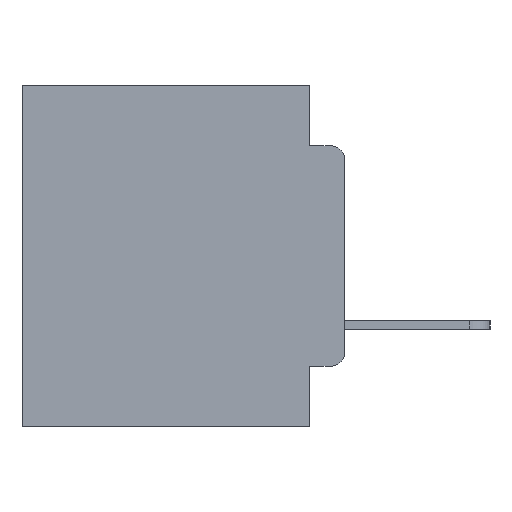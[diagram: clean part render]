
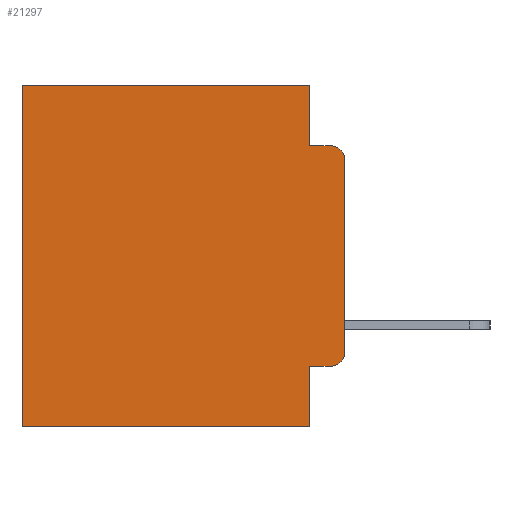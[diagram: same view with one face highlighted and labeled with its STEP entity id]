
A CAD part, left-side view. The second image highlights one B-rep face of the part: STEP entity #21297.
In plain terms, the highlighted planar face has unit normal (-1, 0, 0).
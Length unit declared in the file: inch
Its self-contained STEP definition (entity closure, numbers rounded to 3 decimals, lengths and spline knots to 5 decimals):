
#231 = DIRECTION ( 'NONE',  ( 0., 1., 0. ) ) ;
#335 = ORIENTED_EDGE ( 'NONE', *, *, #5590, .F. ) ;
#476 = VECTOR ( 'NONE', #7063, 39.37008 ) ;
#842 = VERTEX_POINT ( 'NONE', #13256 ) ;
#956 = VECTOR ( 'NONE', #26244, 39.37008 ) ;
#1646 = LINE ( 'NONE', #15390, #10868 ) ;
#1993 = VERTEX_POINT ( 'NONE', #24854 ) ;
#2411 = DIRECTION ( 'NONE',  ( -1., 0., 0. ) ) ;
#2981 = CIRCLE ( 'NONE', #24995, 0.02 ) ;
#3426 = DIRECTION ( 'NONE',  ( 1., 0., 0. ) ) ;
#3777 = CARTESIAN_POINT ( 'NONE',  ( 0.298, 0.02, -0.1085 ) ) ;
#4353 = CARTESIAN_POINT ( 'NONE',  ( 0.298, 0.051, -0.4115 ) ) ;
#4535 = LINE ( 'NONE', #24744, #9102 ) ;
#4929 = CARTESIAN_POINT ( 'NONE',  ( 0.298, 0.051, 0. ) ) ;
#5284 = ORIENTED_EDGE ( 'NONE', *, *, #26712, .T. ) ;
#5350 = LINE ( 'NONE', #10343, #20196 ) ;
#5549 = ORIENTED_EDGE ( 'NONE', *, *, #22947, .T. ) ;
#5590 = EDGE_CURVE ( 'NONE', #842, #29036, #24272, .T. ) ;
#6640 = FACE_OUTER_BOUND ( 'NONE', #8624, .T. ) ;
#6986 = ORIENTED_EDGE ( 'NONE', *, *, #18214, .F. ) ;
#7063 = DIRECTION ( 'NONE',  ( 0., 0., -1. ) ) ;
#7308 = ORIENTED_EDGE ( 'NONE', *, *, #20765, .T. ) ;
#7462 = VECTOR ( 'NONE', #9378, 39.37008 ) ;
#7862 = EDGE_CURVE ( 'NONE', #10213, #24569, #27596, .T. ) ;
#8111 = AXIS2_PLACEMENT_3D ( 'NONE', #20575, #2411, #24910 ) ;
#8624 = EDGE_LOOP ( 'NONE', ( #14654, #5549, #335, #27455, #5284, #23179, #21137, #6986, #7308, #28510 ) ) ;
#9102 = VECTOR ( 'NONE', #27571, 39.37008 ) ;
#9378 = DIRECTION ( 'NONE',  ( 0., 0., -1. ) ) ;
#10139 = CARTESIAN_POINT ( 'NONE',  ( 0.298, 0., 0. ) ) ;
#10213 = VERTEX_POINT ( 'NONE', #28214 ) ;
#10343 = CARTESIAN_POINT ( 'NONE',  ( 0.298, 0., -0.5 ) ) ;
#10488 = CARTESIAN_POINT ( 'NONE',  ( 0.298, 0.02, -0.0885 ) ) ;
#10587 = DIRECTION ( 'NONE',  ( -1., 0., 0. ) ) ;
#10801 = CARTESIAN_POINT ( 'NONE',  ( 0.298, 0.051, 0. ) ) ;
#10868 = VECTOR ( 'NONE', #26693, 39.37008 ) ;
#11604 = VERTEX_POINT ( 'NONE', #4353 ) ;
#13084 = EDGE_CURVE ( 'NONE', #14661, #842, #4535, .T. ) ;
#13256 = CARTESIAN_POINT ( 'NONE',  ( 0.298, 0.051, -0.0885 ) ) ;
#13297 = DIRECTION ( 'NONE',  ( 0., 0., -1. ) ) ;
#14654 = ORIENTED_EDGE ( 'NONE', *, *, #24735, .F. ) ;
#14661 = VERTEX_POINT ( 'NONE', #10801 ) ;
#15390 = CARTESIAN_POINT ( 'NONE',  ( 0.298, 0.051, -0.4115 ) ) ;
#16493 = EDGE_CURVE ( 'NONE', #24280, #1993, #28730, .T. ) ;
#17251 = AXIS2_PLACEMENT_3D ( 'NONE', #10139, #3426, #13297 ) ;
#17669 = VERTEX_POINT ( 'NONE', #21399 ) ;
#18214 = EDGE_CURVE ( 'NONE', #11604, #21427, #28245, .T. ) ;
#19735 = DIRECTION ( 'NONE',  ( 0., 0., -1. ) ) ;
#20196 = VECTOR ( 'NONE', #21965, 39.37008 ) ;
#20575 = CARTESIAN_POINT ( 'NONE',  ( 0.298, 0.02, -0.3915 ) ) ;
#20765 = EDGE_CURVE ( 'NONE', #11604, #10213, #1646, .T. ) ;
#21137 = ORIENTED_EDGE ( 'NONE', *, *, #24698, .F. ) ;
#21297 = ADVANCED_FACE ( 'NONE', ( #6640 ), #23628, .F. ) ;
#21381 = CARTESIAN_POINT ( 'NONE',  ( 0.298, 0.473, 0. ) ) ;
#21399 = CARTESIAN_POINT ( 'NONE',  ( 0.298, 0., -0.1085 ) ) ;
#21427 = VERTEX_POINT ( 'NONE', #25463 ) ;
#21949 = VECTOR ( 'NONE', #26487, 39.37008 ) ;
#21965 = DIRECTION ( 'NONE',  ( 0., 1., 0. ) ) ;
#22063 = CARTESIAN_POINT ( 'NONE',  ( 0.298, 0., 0. ) ) ;
#22947 = EDGE_CURVE ( 'NONE', #17669, #29036, #2981, .T. ) ;
#23179 = ORIENTED_EDGE ( 'NONE', *, *, #16493, .T. ) ;
#23628 = PLANE ( 'NONE',  #17251 ) ;
#24272 = LINE ( 'NONE', #28393, #956 ) ;
#24280 = VERTEX_POINT ( 'NONE', #21381 ) ;
#24569 = VERTEX_POINT ( 'NONE', #28527 ) ;
#24698 = EDGE_CURVE ( 'NONE', #21427, #1993, #5350, .T. ) ;
#24735 = EDGE_CURVE ( 'NONE', #17669, #24569, #25800, .T. ) ;
#24744 = CARTESIAN_POINT ( 'NONE',  ( 0.298, 0.051, 0. ) ) ;
#24854 = CARTESIAN_POINT ( 'NONE',  ( 0.298, 0.473, -0.5 ) ) ;
#24910 = DIRECTION ( 'NONE',  ( 0., 0., -1. ) ) ;
#24994 = CARTESIAN_POINT ( 'NONE',  ( 0.298, 0., 0. ) ) ;
#24995 = AXIS2_PLACEMENT_3D ( 'NONE', #3777, #10587, #19735 ) ;
#25463 = CARTESIAN_POINT ( 'NONE',  ( 0.298, 0.051, -0.5 ) ) ;
#25800 = LINE ( 'NONE', #22063, #21949 ) ;
#26244 = DIRECTION ( 'NONE',  ( 0., -1., 0. ) ) ;
#26389 = VECTOR ( 'NONE', #231, 39.37008 ) ;
#26487 = DIRECTION ( 'NONE',  ( 0., 0., -1. ) ) ;
#26693 = DIRECTION ( 'NONE',  ( 0., -1., 0. ) ) ;
#26712 = EDGE_CURVE ( 'NONE', #14661, #24280, #28136, .T. ) ;
#27125 = CARTESIAN_POINT ( 'NONE',  ( 0.298, 0.473, 0. ) ) ;
#27455 = ORIENTED_EDGE ( 'NONE', *, *, #13084, .F. ) ;
#27571 = DIRECTION ( 'NONE',  ( 0., 0., -1. ) ) ;
#27596 = CIRCLE ( 'NONE', #8111, 0.02 ) ;
#28136 = LINE ( 'NONE', #24994, #26389 ) ;
#28214 = CARTESIAN_POINT ( 'NONE',  ( 0.298, 0.02, -0.4115 ) ) ;
#28245 = LINE ( 'NONE', #4929, #7462 ) ;
#28393 = CARTESIAN_POINT ( 'NONE',  ( 0.298, 0.051, -0.0885 ) ) ;
#28510 = ORIENTED_EDGE ( 'NONE', *, *, #7862, .T. ) ;
#28527 = CARTESIAN_POINT ( 'NONE',  ( 0.298, 0., -0.3915 ) ) ;
#28730 = LINE ( 'NONE', #27125, #476 ) ;
#29036 = VERTEX_POINT ( 'NONE', #10488 ) ;
